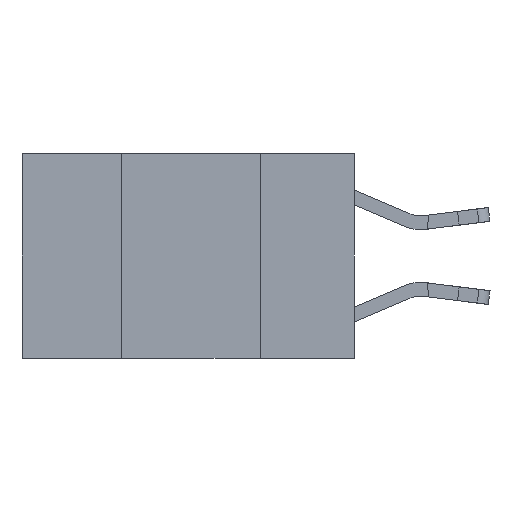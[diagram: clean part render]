
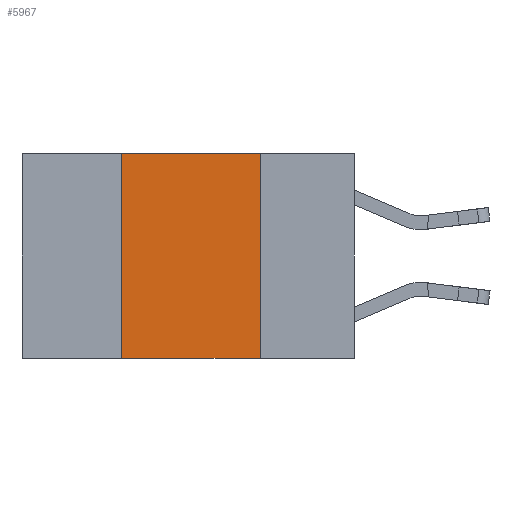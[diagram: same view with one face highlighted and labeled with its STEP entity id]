
A CAD part, left-side view. The second image highlights one B-rep face of the part: STEP entity #5967.
In plain terms, the highlighted planar face has unit normal (-1, 0, 0).
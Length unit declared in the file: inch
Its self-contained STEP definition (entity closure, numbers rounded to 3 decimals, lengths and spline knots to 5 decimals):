
#387 = EDGE_CURVE ( 'NONE', #23034, #11682, #16063, .T. ) ;
#1236 = VERTEX_POINT ( 'NONE', #11178 ) ;
#1731 = VECTOR ( 'NONE', #19461, 39.37008 ) ;
#2226 = CARTESIAN_POINT ( 'NONE',  ( 0., 0.42, 0. ) ) ;
#2960 = CARTESIAN_POINT ( 'NONE',  ( 0., 0.17, 0. ) ) ;
#4560 = PLANE ( 'NONE',  #13543 ) ;
#5402 = FACE_OUTER_BOUND ( 'NONE', #8181, .T. ) ;
#5815 = CARTESIAN_POINT ( 'NONE',  ( 0., 0.17, -0.37 ) ) ;
#5967 = ADVANCED_FACE ( 'NONE', ( #5402 ), #4560, .F. ) ;
#7868 = DIRECTION ( 'NONE',  ( 0., 0., 1. ) ) ;
#8181 = EDGE_LOOP ( 'NONE', ( #12502, #20139, #10111, #14731 ) ) ;
#8230 = CARTESIAN_POINT ( 'NONE',  ( 0., 0.6, 0. ) ) ;
#8252 = CARTESIAN_POINT ( 'NONE',  ( 0., 0.42, 0. ) ) ;
#8342 = DIRECTION ( 'NONE',  ( 0., 0., -1. ) ) ;
#8962 = VECTOR ( 'NONE', #23975, 39.37008 ) ;
#10111 = ORIENTED_EDGE ( 'NONE', *, *, #15936, .F. ) ;
#10924 = EDGE_CURVE ( 'NONE', #1236, #11682, #18943, .T. ) ;
#11094 = VECTOR ( 'NONE', #15607, 39.37008 ) ;
#11178 = CARTESIAN_POINT ( 'NONE',  ( 0., 0.42, -0.37 ) ) ;
#11682 = VERTEX_POINT ( 'NONE', #5815 ) ;
#11700 = LINE ( 'NONE', #8230, #1731 ) ;
#12502 = ORIENTED_EDGE ( 'NONE', *, *, #387, .F. ) ;
#12627 = VERTEX_POINT ( 'NONE', #8252 ) ;
#13543 = AXIS2_PLACEMENT_3D ( 'NONE', #17702, #19582, #8342 ) ;
#14308 = LINE ( 'NONE', #2226, #23696 ) ;
#14565 = CARTESIAN_POINT ( 'NONE',  ( 0., 0.6, -0.37 ) ) ;
#14731 = ORIENTED_EDGE ( 'NONE', *, *, #10924, .T. ) ;
#15371 = EDGE_CURVE ( 'NONE', #12627, #23034, #11700, .T. ) ;
#15607 = DIRECTION ( 'NONE',  ( 0., 0., -1. ) ) ;
#15734 = CARTESIAN_POINT ( 'NONE',  ( 0., 0.17, 0. ) ) ;
#15936 = EDGE_CURVE ( 'NONE', #1236, #12627, #14308, .T. ) ;
#16063 = LINE ( 'NONE', #15734, #11094 ) ;
#17702 = CARTESIAN_POINT ( 'NONE',  ( 0., 0.6, 0. ) ) ;
#18943 = LINE ( 'NONE', #14565, #8962 ) ;
#19461 = DIRECTION ( 'NONE',  ( 0., -1., 0. ) ) ;
#19582 = DIRECTION ( 'NONE',  ( 1., 0., 0. ) ) ;
#20139 = ORIENTED_EDGE ( 'NONE', *, *, #15371, .F. ) ;
#23034 = VERTEX_POINT ( 'NONE', #2960 ) ;
#23696 = VECTOR ( 'NONE', #7868, 39.37008 ) ;
#23975 = DIRECTION ( 'NONE',  ( 0., -1., 0. ) ) ;
